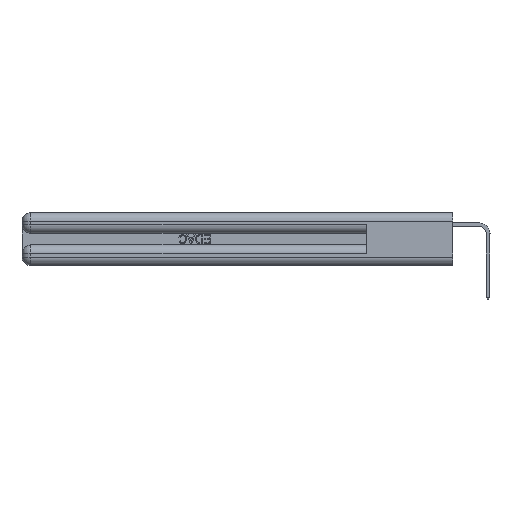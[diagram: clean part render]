
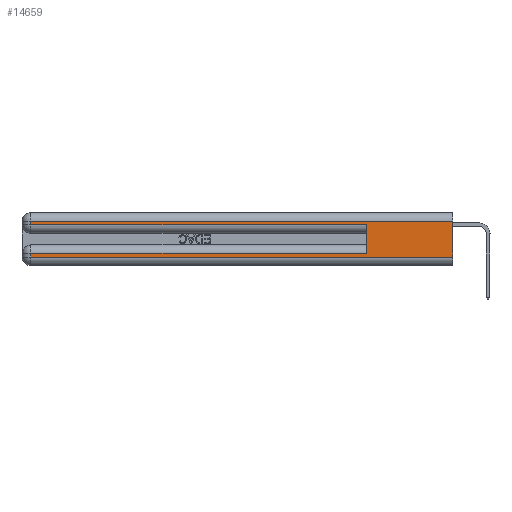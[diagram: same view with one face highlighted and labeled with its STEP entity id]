
A CAD part, left-side view. The second image highlights one B-rep face of the part: STEP entity #14659.
In plain terms, the highlighted planar face has unit normal (-1, 0, 0).
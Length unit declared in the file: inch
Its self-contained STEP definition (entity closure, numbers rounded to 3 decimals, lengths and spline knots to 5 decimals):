
#84 = ORIENTED_EDGE ( 'NONE', *, *, #10081, .T. ) ;
#1723 = VECTOR ( 'NONE', #38926, 39.37008 ) ;
#1745 = VERTEX_POINT ( 'NONE', #5351 ) ;
#2006 = VECTOR ( 'NONE', #13648, 39.37008 ) ;
#2378 = VECTOR ( 'NONE', #24270, 39.37008 ) ;
#2500 = DIRECTION ( 'NONE',  ( 0., 0., -1. ) ) ;
#3025 = LINE ( 'NONE', #7096, #2006 ) ;
#4011 = VERTEX_POINT ( 'NONE', #28973 ) ;
#5351 = CARTESIAN_POINT ( 'NONE',  ( 0., 2.94, 0.31 ) ) ;
#5588 = LINE ( 'NONE', #40657, #6612 ) ;
#5907 = DIRECTION ( 'NONE',  ( 0., 0., -1. ) ) ;
#6109 = CARTESIAN_POINT ( 'NONE',  ( 0., 2.94, 0.37 ) ) ;
#6612 = VECTOR ( 'NONE', #24239, 39.37008 ) ;
#6690 = DIRECTION ( 'NONE',  ( 0., -1., 0. ) ) ;
#6719 = ORIENTED_EDGE ( 'NONE', *, *, #24572, .T. ) ;
#6808 = VERTEX_POINT ( 'NONE', #28824 ) ;
#7096 = CARTESIAN_POINT ( 'NONE',  ( 0., 0., 0.085 ) ) ;
#9953 = EDGE_CURVE ( 'NONE', #21972, #24316, #11735, .T. ) ;
#10008 = LINE ( 'NONE', #34100, #2378 ) ;
#10081 = EDGE_CURVE ( 'NONE', #6808, #1745, #5588, .T. ) ;
#11735 = LINE ( 'NONE', #29551, #37901 ) ;
#12177 = CARTESIAN_POINT ( 'NONE',  ( 0., 2.94, 0.37 ) ) ;
#12815 = EDGE_LOOP ( 'NONE', ( #14165, #84, #39996, #15485, #37336, #6719, #27062, #41839 ) ) ;
#13648 = DIRECTION ( 'NONE',  ( 0., 1., 0. ) ) ;
#14165 = ORIENTED_EDGE ( 'NONE', *, *, #29161, .F. ) ;
#14659 = ADVANCED_FACE ( 'NONE', ( #23592 ), #22158, .F. ) ;
#15485 = ORIENTED_EDGE ( 'NONE', *, *, #9953, .T. ) ;
#17701 = VECTOR ( 'NONE', #2500, 39.37008 ) ;
#18544 = VERTEX_POINT ( 'NONE', #29203 ) ;
#19029 = LINE ( 'NONE', #6109, #1723 ) ;
#19277 = CARTESIAN_POINT ( 'NONE',  ( 0., 0., 0.37 ) ) ;
#21972 = VERTEX_POINT ( 'NONE', #39364 ) ;
#22158 = PLANE ( 'NONE',  #32219 ) ;
#22560 = DIRECTION ( 'NONE',  ( 0., 0., -1. ) ) ;
#23244 = LINE ( 'NONE', #32601, #40756 ) ;
#23592 = FACE_OUTER_BOUND ( 'NONE', #12815, .T. ) ;
#23656 = VERTEX_POINT ( 'NONE', #41115 ) ;
#24239 = DIRECTION ( 'NONE',  ( 0., 1., 0. ) ) ;
#24270 = DIRECTION ( 'NONE',  ( 0., 0., 1. ) ) ;
#24316 = VERTEX_POINT ( 'NONE', #28660 ) ;
#24572 = EDGE_CURVE ( 'NONE', #23656, #30590, #3025, .T. ) ;
#25450 = DIRECTION ( 'NONE',  ( 1., 0., 0. ) ) ;
#25477 = EDGE_CURVE ( 'NONE', #30590, #4011, #19029, .T. ) ;
#25963 = DIRECTION ( 'NONE',  ( 0., -1., 0. ) ) ;
#27062 = ORIENTED_EDGE ( 'NONE', *, *, #25477, .T. ) ;
#28660 = CARTESIAN_POINT ( 'NONE',  ( 0., 0.6, 0.285 ) ) ;
#28824 = CARTESIAN_POINT ( 'NONE',  ( 0., 0., 0.31 ) ) ;
#28973 = CARTESIAN_POINT ( 'NONE',  ( 0., 2.94, 0.06 ) ) ;
#29030 = EDGE_CURVE ( 'NONE', #1745, #21972, #29488, .T. ) ;
#29161 = EDGE_CURVE ( 'NONE', #6808, #18544, #32059, .T. ) ;
#29203 = CARTESIAN_POINT ( 'NONE',  ( 0., 0., 0.06 ) ) ;
#29488 = LINE ( 'NONE', #12177, #17701 ) ;
#29502 = EDGE_CURVE ( 'NONE', #23656, #24316, #10008, .T. ) ;
#29551 = CARTESIAN_POINT ( 'NONE',  ( 0., 0., 0.285 ) ) ;
#30590 = VERTEX_POINT ( 'NONE', #33446 ) ;
#32059 = LINE ( 'NONE', #19277, #39801 ) ;
#32219 = AXIS2_PLACEMENT_3D ( 'NONE', #35292, #25450, #5907 ) ;
#32601 = CARTESIAN_POINT ( 'NONE',  ( 0., 0., 0.06 ) ) ;
#33446 = CARTESIAN_POINT ( 'NONE',  ( 0., 2.94, 0.085 ) ) ;
#34100 = CARTESIAN_POINT ( 'NONE',  ( 0., 0.6, 0.145 ) ) ;
#35292 = CARTESIAN_POINT ( 'NONE',  ( 0., 0., 0.37 ) ) ;
#35812 = EDGE_CURVE ( 'NONE', #4011, #18544, #23244, .T. ) ;
#37336 = ORIENTED_EDGE ( 'NONE', *, *, #29502, .F. ) ;
#37901 = VECTOR ( 'NONE', #6690, 39.37008 ) ;
#38926 = DIRECTION ( 'NONE',  ( 0., 0., -1. ) ) ;
#39364 = CARTESIAN_POINT ( 'NONE',  ( 0., 2.94, 0.285 ) ) ;
#39801 = VECTOR ( 'NONE', #22560, 39.37008 ) ;
#39996 = ORIENTED_EDGE ( 'NONE', *, *, #29030, .T. ) ;
#40657 = CARTESIAN_POINT ( 'NONE',  ( 0., 0., 0.31 ) ) ;
#40756 = VECTOR ( 'NONE', #25963, 39.37008 ) ;
#41115 = CARTESIAN_POINT ( 'NONE',  ( 0., 0.6, 0.085 ) ) ;
#41839 = ORIENTED_EDGE ( 'NONE', *, *, #35812, .T. ) ;
